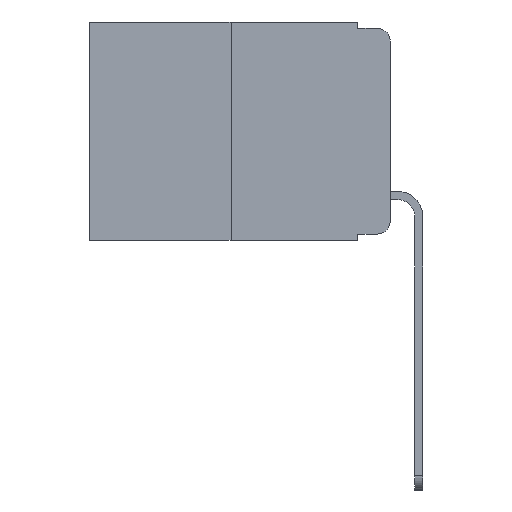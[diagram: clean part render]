
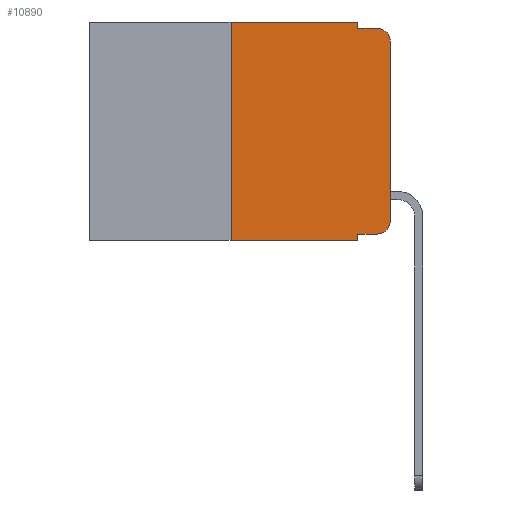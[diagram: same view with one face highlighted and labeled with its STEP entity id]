
A CAD part, left-side view. The second image highlights one B-rep face of the part: STEP entity #10890.
In plain terms, the highlighted planar face has unit normal (-1, 0, 0).
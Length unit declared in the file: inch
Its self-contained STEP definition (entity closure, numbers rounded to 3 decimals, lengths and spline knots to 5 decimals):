
#386 = DIRECTION ( 'NONE',  ( 0., -1., 0. ) ) ;
#705 = CARTESIAN_POINT ( 'NONE',  ( 0., 0.02, -0.313 ) ) ;
#1060 = EDGE_CURVE ( 'NONE', #16632, #7795, #21169, .T. ) ;
#1236 = CARTESIAN_POINT ( 'NONE',  ( 0., 0.02, -0.333 ) ) ;
#1437 = EDGE_CURVE ( 'NONE', #5040, #16632, #7687, .T. ) ;
#2053 = CARTESIAN_POINT ( 'NONE',  ( 0., 0., -0.03 ) ) ;
#2136 = CARTESIAN_POINT ( 'NONE',  ( 0., 0.051, -0.343 ) ) ;
#2546 = LINE ( 'NONE', #18686, #7103 ) ;
#2872 = VECTOR ( 'NONE', #20510, 39.37008 ) ;
#3587 = DIRECTION ( 'NONE',  ( 0., 0., -1. ) ) ;
#3743 = PLANE ( 'NONE',  #3877 ) ;
#3840 = VECTOR ( 'NONE', #5470, 39.37008 ) ;
#3877 = AXIS2_PLACEMENT_3D ( 'NONE', #16989, #24668, #3587 ) ;
#4318 = DIRECTION ( 'NONE',  ( -1., 0., 0. ) ) ;
#4661 = VECTOR ( 'NONE', #386, 39.37008 ) ;
#4693 = AXIS2_PLACEMENT_3D ( 'NONE', #705, #4318, #21492 ) ;
#4696 = CARTESIAN_POINT ( 'NONE',  ( 0., 0.051, -0.333 ) ) ;
#5040 = VERTEX_POINT ( 'NONE', #17810 ) ;
#5470 = DIRECTION ( 'NONE',  ( 0., 0., 1. ) ) ;
#5600 = ORIENTED_EDGE ( 'NONE', *, *, #24491, .F. ) ;
#5870 = VERTEX_POINT ( 'NONE', #16270 ) ;
#5999 = VECTOR ( 'NONE', #12961, 39.37008 ) ;
#6022 = CIRCLE ( 'NONE', #11978, 0.02 ) ;
#6101 = LINE ( 'NONE', #23492, #14789 ) ;
#6332 = ORIENTED_EDGE ( 'NONE', *, *, #14517, .T. ) ;
#7095 = EDGE_CURVE ( 'NONE', #11960, #24301, #8064, .T. ) ;
#7103 = VECTOR ( 'NONE', #20742, 39.37008 ) ;
#7262 = ORIENTED_EDGE ( 'NONE', *, *, #14045, .T. ) ;
#7313 = FACE_OUTER_BOUND ( 'NONE', #18391, .T. ) ;
#7687 = LINE ( 'NONE', #22449, #2872 ) ;
#7703 = ORIENTED_EDGE ( 'NONE', *, *, #19529, .F. ) ;
#7795 = VERTEX_POINT ( 'NONE', #12338 ) ;
#8064 = LINE ( 'NONE', #24311, #3840 ) ;
#8253 = DIRECTION ( 'NONE',  ( 0., 0., -1. ) ) ;
#9296 = EDGE_CURVE ( 'NONE', #5870, #10938, #2546, .T. ) ;
#9776 = LINE ( 'NONE', #21405, #4661 ) ;
#10890 = ADVANCED_FACE ( 'NONE', ( #7313 ), #3743, .F. ) ;
#10938 = VERTEX_POINT ( 'NONE', #14915 ) ;
#11096 = EDGE_CURVE ( 'NONE', #18263, #11960, #16281, .T. ) ;
#11107 = LINE ( 'NONE', #18559, #5999 ) ;
#11960 = VERTEX_POINT ( 'NONE', #18781 ) ;
#11978 = AXIS2_PLACEMENT_3D ( 'NONE', #15469, #15301, #15222 ) ;
#12338 = CARTESIAN_POINT ( 'NONE',  ( 0., 0.02, -0.01 ) ) ;
#12873 = VERTEX_POINT ( 'NONE', #2136 ) ;
#12951 = ORIENTED_EDGE ( 'NONE', *, *, #9296, .F. ) ;
#12961 = DIRECTION ( 'NONE',  ( 0., -1., 0. ) ) ;
#14045 = EDGE_CURVE ( 'NONE', #24301, #7795, #6022, .T. ) ;
#14069 = ORIENTED_EDGE ( 'NONE', *, *, #1437, .F. ) ;
#14134 = LINE ( 'NONE', #16513, #15310 ) ;
#14517 = EDGE_CURVE ( 'NONE', #5870, #12873, #11107, .T. ) ;
#14789 = VECTOR ( 'NONE', #17912, 39.37008 ) ;
#14915 = CARTESIAN_POINT ( 'NONE',  ( 0., 0.25, 0. ) ) ;
#15222 = DIRECTION ( 'NONE',  ( 0., 0., -1. ) ) ;
#15301 = DIRECTION ( 'NONE',  ( -1., 0., 0. ) ) ;
#15310 = VECTOR ( 'NONE', #8253, 39.37008 ) ;
#15469 = CARTESIAN_POINT ( 'NONE',  ( 0., 0.02, -0.03 ) ) ;
#16270 = CARTESIAN_POINT ( 'NONE',  ( 0., 0.25, -0.343 ) ) ;
#16281 = CIRCLE ( 'NONE', #4693, 0.02 ) ;
#16513 = CARTESIAN_POINT ( 'NONE',  ( 0., 0.051, 0. ) ) ;
#16632 = VERTEX_POINT ( 'NONE', #19007 ) ;
#16989 = CARTESIAN_POINT ( 'NONE',  ( 0., 0.473, 0. ) ) ;
#17614 = CARTESIAN_POINT ( 'NONE',  ( 0., 0.051, -0.01 ) ) ;
#17810 = CARTESIAN_POINT ( 'NONE',  ( 0., 0.051, 0. ) ) ;
#17912 = DIRECTION ( 'NONE',  ( 0., -1., 0. ) ) ;
#18263 = VERTEX_POINT ( 'NONE', #1236 ) ;
#18391 = EDGE_LOOP ( 'NONE', ( #24726, #7262, #23444, #14069, #5600, #12951, #6332, #7703, #18969, #20756 ) ) ;
#18559 = CARTESIAN_POINT ( 'NONE',  ( 0., 0.473, -0.343 ) ) ;
#18686 = CARTESIAN_POINT ( 'NONE',  ( 0., 0.25, 0. ) ) ;
#18781 = CARTESIAN_POINT ( 'NONE',  ( 0., 0., -0.313 ) ) ;
#18969 = ORIENTED_EDGE ( 'NONE', *, *, #22713, .T. ) ;
#19007 = CARTESIAN_POINT ( 'NONE',  ( 0., 0.051, -0.01 ) ) ;
#19446 = DIRECTION ( 'NONE',  ( 0., -1., 0. ) ) ;
#19529 = EDGE_CURVE ( 'NONE', #21176, #12873, #14134, .T. ) ;
#20510 = DIRECTION ( 'NONE',  ( 0., 0., -1. ) ) ;
#20742 = DIRECTION ( 'NONE',  ( 0., 0., 1. ) ) ;
#20756 = ORIENTED_EDGE ( 'NONE', *, *, #11096, .T. ) ;
#21169 = LINE ( 'NONE', #17614, #24468 ) ;
#21176 = VERTEX_POINT ( 'NONE', #4696 ) ;
#21405 = CARTESIAN_POINT ( 'NONE',  ( 0., 0.051, -0.333 ) ) ;
#21492 = DIRECTION ( 'NONE',  ( 0., 0., -1. ) ) ;
#22449 = CARTESIAN_POINT ( 'NONE',  ( 0., 0.051, 0. ) ) ;
#22713 = EDGE_CURVE ( 'NONE', #21176, #18263, #9776, .T. ) ;
#23444 = ORIENTED_EDGE ( 'NONE', *, *, #1060, .F. ) ;
#23492 = CARTESIAN_POINT ( 'NONE',  ( 0., 0.473, 0. ) ) ;
#24301 = VERTEX_POINT ( 'NONE', #2053 ) ;
#24311 = CARTESIAN_POINT ( 'NONE',  ( 0., 0., 0. ) ) ;
#24468 = VECTOR ( 'NONE', #19446, 39.37008 ) ;
#24491 = EDGE_CURVE ( 'NONE', #10938, #5040, #6101, .T. ) ;
#24668 = DIRECTION ( 'NONE',  ( 1., 0., 0. ) ) ;
#24726 = ORIENTED_EDGE ( 'NONE', *, *, #7095, .T. ) ;
